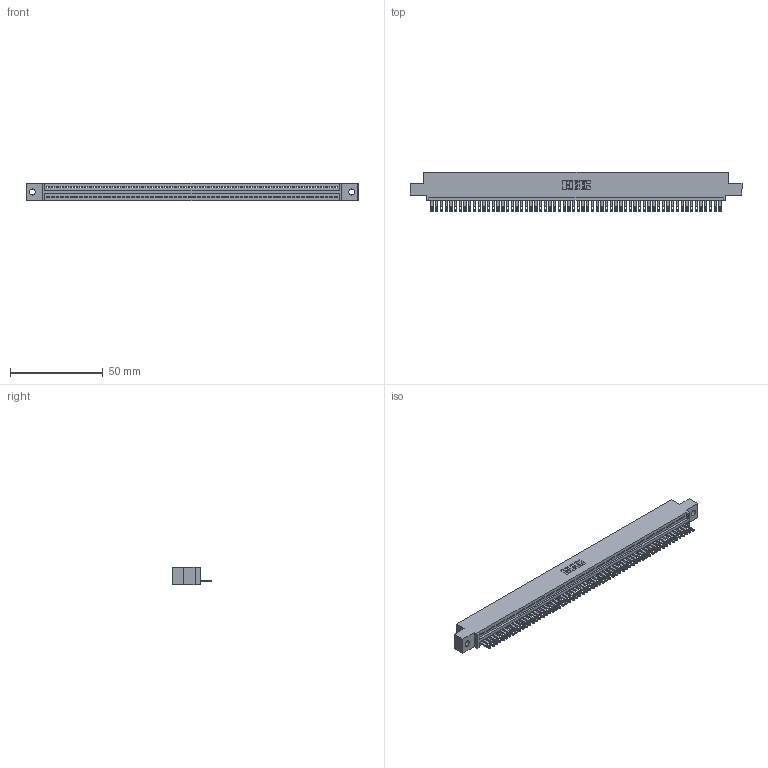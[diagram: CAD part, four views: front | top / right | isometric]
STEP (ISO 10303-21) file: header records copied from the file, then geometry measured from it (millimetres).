
FILE_DESCRIPTION (( 'STEP AP203' ), '1' );
FILE_NAME ('345-062-500-402.STEP', '2018-09-27T10:31:49', ( '' ), ( '' ), 'SwSTEP 2.0', 'SolidWorks 2016', '' );
FILE_SCHEMA (( 'CONFIG_CONTROL_DESIGN' ));
Length unit declared in the file: inch
Products named in the file (3): 345-062-500-402; 345-292-001_345-293-100; 345 Part_0.110 Offset - 0.128 Dia
Assembly tree (63 placements, depth 2):
  345-062-500-402
    345 Part_0.110 Offset - 0.128 Dia
    345-292-001_345-293-100  x62
Bounding box: 178.69 x 21.51 x 9.4 mm (x, y, z)
Volume: 17064.2 mm3; surface area: 22898.2 mm2
Topology: 63 solids, 63 shells, 3478 faces, 10769 edges, 7178 vertices
Faces by surface type: plane 2192, cylinder 1286
Entity records: 44035 total; most frequent: CARTESIAN_POINT 7634, ORIENTED_EDGE 7630, DIRECTION 6639, EDGE_CURVE 3815, VECTOR 3431, LINE 3431, VERTEX_POINT 2542, AXIS2_PLACEMENT_3D 1604
